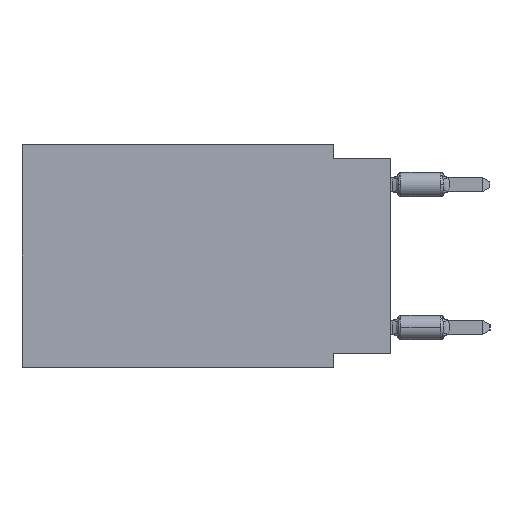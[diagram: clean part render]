
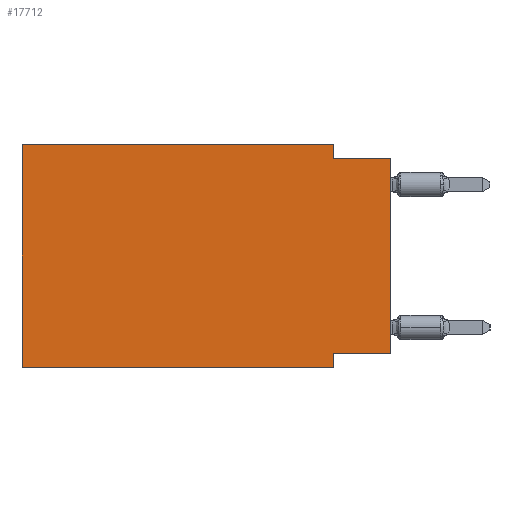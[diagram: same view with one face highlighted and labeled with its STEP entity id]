
A CAD part, left-side view. The second image highlights one B-rep face of the part: STEP entity #17712.
In plain terms, the highlighted planar face has unit normal (-1, 0, 0).
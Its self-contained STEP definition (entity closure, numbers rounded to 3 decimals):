
#734 = CARTESIAN_POINT ( 'NONE',  ( 0., 0., -9.271 ) ) ;
#759 = VERTEX_POINT ( 'NONE', #38609 ) ;
#890 = EDGE_CURVE ( 'NONE', #35987, #40052, #14242, .T. ) ;
#1213 = VECTOR ( 'NONE', #31976, 1000. ) ;
#1979 = VERTEX_POINT ( 'NONE', #34382 ) ;
#2056 = DIRECTION ( 'NONE',  ( 0., 0., -1. ) ) ;
#3047 = CARTESIAN_POINT ( 'NONE',  ( 0., 0., 0. ) ) ;
#4957 = LINE ( 'NONE', #12529, #22012 ) ;
#5080 = VERTEX_POINT ( 'NONE', #40772 ) ;
#5620 = CARTESIAN_POINT ( 'NONE',  ( 0., 16.383, 0. ) ) ;
#6382 = EDGE_LOOP ( 'NONE', ( #21020, #17045, #37500, #46131, #13879, #19624, #32354, #24307 ) ) ;
#6620 = EDGE_CURVE ( 'NONE', #11605, #29625, #4957, .T. ) ;
#8236 = EDGE_CURVE ( 'NONE', #759, #40052, #44648, .T. ) ;
#11605 = VERTEX_POINT ( 'NONE', #28696 ) ;
#11949 = AXIS2_PLACEMENT_3D ( 'NONE', #5620, #31636, #46074 ) ;
#11976 = CARTESIAN_POINT ( 'NONE',  ( 0., 2.54, 0. ) ) ;
#12082 = LINE ( 'NONE', #734, #25290 ) ;
#12529 = CARTESIAN_POINT ( 'NONE',  ( 0., 16.383, 0. ) ) ;
#13879 = ORIENTED_EDGE ( 'NONE', *, *, #29466, .F. ) ;
#14242 = LINE ( 'NONE', #18010, #26975 ) ;
#14482 = VECTOR ( 'NONE', #15655, 1000. ) ;
#14690 = VECTOR ( 'NONE', #23307, 1000. ) ;
#15514 = LINE ( 'NONE', #11976, #14690 ) ;
#15633 = DIRECTION ( 'NONE',  ( 0., 1., 0. ) ) ;
#15655 = DIRECTION ( 'NONE',  ( 0., -1., 0. ) ) ;
#15994 = CARTESIAN_POINT ( 'NONE',  ( 0., 2.54, -9.906 ) ) ;
#17045 = ORIENTED_EDGE ( 'NONE', *, *, #42854, .F. ) ;
#17416 = VECTOR ( 'NONE', #2056, 1000. ) ;
#17712 = ADVANCED_FACE ( 'NONE', ( #27858 ), #42308, .F. ) ;
#18010 = CARTESIAN_POINT ( 'NONE',  ( 0., 16.383, -9.906 ) ) ;
#19624 = ORIENTED_EDGE ( 'NONE', *, *, #890, .T. ) ;
#21020 = ORIENTED_EDGE ( 'NONE', *, *, #40127, .T. ) ;
#21084 = CARTESIAN_POINT ( 'NONE',  ( 0., 16.383, 0. ) ) ;
#21599 = CARTESIAN_POINT ( 'NONE',  ( 0., 0., -9.271 ) ) ;
#22012 = VECTOR ( 'NONE', #40926, 1000. ) ;
#22257 = CARTESIAN_POINT ( 'NONE',  ( 0., 2.54, 0. ) ) ;
#23307 = DIRECTION ( 'NONE',  ( 0., 0., -1. ) ) ;
#24307 = ORIENTED_EDGE ( 'NONE', *, *, #27829, .F. ) ;
#24866 = LINE ( 'NONE', #21084, #1213 ) ;
#25290 = VECTOR ( 'NONE', #15633, 1000. ) ;
#26975 = VECTOR ( 'NONE', #43105, 1000. ) ;
#27068 = EDGE_CURVE ( 'NONE', #29625, #1979, #15514, .T. ) ;
#27829 = EDGE_CURVE ( 'NONE', #34719, #759, #12082, .T. ) ;
#27858 = FACE_OUTER_BOUND ( 'NONE', #6382, .T. ) ;
#28696 = CARTESIAN_POINT ( 'NONE',  ( 0., 16.383, 0. ) ) ;
#29466 = EDGE_CURVE ( 'NONE', #35987, #11605, #24866, .T. ) ;
#29625 = VERTEX_POINT ( 'NONE', #22257 ) ;
#31636 = DIRECTION ( 'NONE',  ( 1., 0., 0. ) ) ;
#31935 = DIRECTION ( 'NONE',  ( 0., 0., 1. ) ) ;
#31976 = DIRECTION ( 'NONE',  ( 0., 0., 1. ) ) ;
#32354 = ORIENTED_EDGE ( 'NONE', *, *, #8236, .F. ) ;
#34382 = CARTESIAN_POINT ( 'NONE',  ( 0., 2.54, -0.635 ) ) ;
#34719 = VERTEX_POINT ( 'NONE', #21599 ) ;
#35464 = LINE ( 'NONE', #3047, #43333 ) ;
#35987 = VERTEX_POINT ( 'NONE', #43622 ) ;
#37500 = ORIENTED_EDGE ( 'NONE', *, *, #27068, .F. ) ;
#38609 = CARTESIAN_POINT ( 'NONE',  ( 0., 2.54, -9.271 ) ) ;
#40052 = VERTEX_POINT ( 'NONE', #46622 ) ;
#40127 = EDGE_CURVE ( 'NONE', #34719, #5080, #35464, .T. ) ;
#40772 = CARTESIAN_POINT ( 'NONE',  ( 0., 0., -0.635 ) ) ;
#40926 = DIRECTION ( 'NONE',  ( 0., -1., 0. ) ) ;
#42308 = PLANE ( 'NONE',  #11949 ) ;
#42854 = EDGE_CURVE ( 'NONE', #1979, #5080, #43618, .T. ) ;
#43105 = DIRECTION ( 'NONE',  ( 0., -1., 0. ) ) ;
#43333 = VECTOR ( 'NONE', #31935, 1000. ) ;
#43618 = LINE ( 'NONE', #44065, #14482 ) ;
#43622 = CARTESIAN_POINT ( 'NONE',  ( 0., 16.383, -9.906 ) ) ;
#44065 = CARTESIAN_POINT ( 'NONE',  ( 0., 0., -0.635 ) ) ;
#44648 = LINE ( 'NONE', #15994, #17416 ) ;
#46074 = DIRECTION ( 'NONE',  ( 0., 0., -1. ) ) ;
#46131 = ORIENTED_EDGE ( 'NONE', *, *, #6620, .F. ) ;
#46622 = CARTESIAN_POINT ( 'NONE',  ( 0., 2.54, -9.906 ) ) ;
